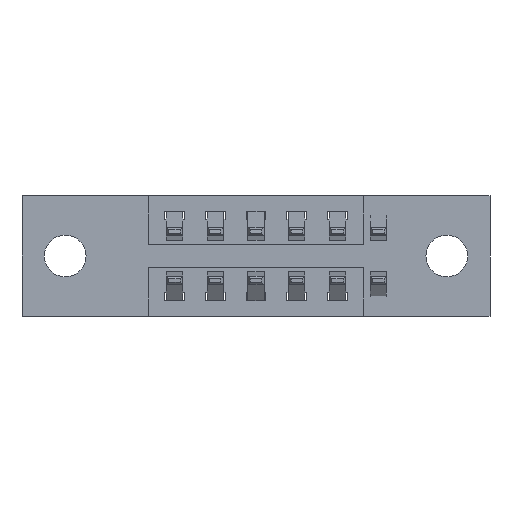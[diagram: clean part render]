
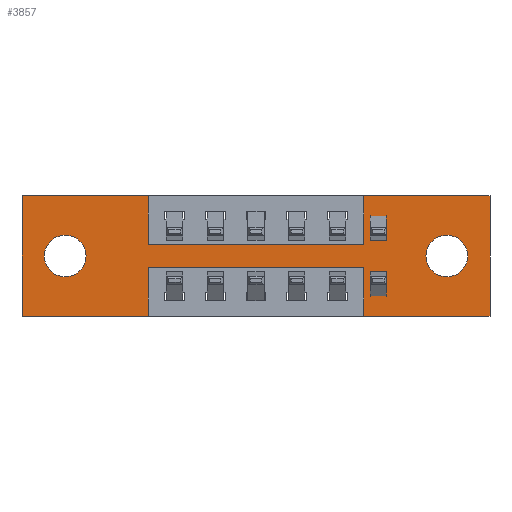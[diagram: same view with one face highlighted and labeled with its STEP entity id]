
A CAD part, front view. The second image highlights one B-rep face of the part: STEP entity #3857.
In plain terms, the highlighted planar face has unit normal (0, -1, 0).
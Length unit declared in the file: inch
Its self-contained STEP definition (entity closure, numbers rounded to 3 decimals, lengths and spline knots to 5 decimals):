
#3 = AXIS2_PLACEMENT_3D ( 'NONE', #1842, #5162, #1243 ) ;
#109 = ORIENTED_EDGE ( 'NONE', *, *, #1768, .F. ) ;
#117 = EDGE_CURVE ( 'NONE', #2051, #4349, #4844, .T. ) ;
#152 = ORIENTED_EDGE ( 'NONE', *, *, #5313, .T. ) ;
#249 = CARTESIAN_POINT ( 'NONE',  ( 0.3875, 0., -0.22 ) ) ;
#291 = DIRECTION ( 'NONE',  ( 0., 0., -1. ) ) ;
#363 = VECTOR ( 'NONE', #3285, 39.37008 ) ;
#412 = VERTEX_POINT ( 'NONE', #2146 ) ;
#483 = EDGE_CURVE ( 'NONE', #7399, #4806, #1431, .T. ) ;
#634 = ORIENTED_EDGE ( 'NONE', *, *, #5431, .F. ) ;
#654 = CARTESIAN_POINT ( 'NONE',  ( 0.3875, 0., 0. ) ) ;
#701 = VECTOR ( 'NONE', #8024, 39.37008 ) ;
#726 = ORIENTED_EDGE ( 'NONE', *, *, #6611, .F. ) ;
#767 = VECTOR ( 'NONE', #4668, 39.37008 ) ;
#812 = ORIENTED_EDGE ( 'NONE', *, *, #483, .F. ) ;
#901 = VERTEX_POINT ( 'NONE', #5119 ) ;
#937 = FACE_BOUND ( 'NONE', #2978, .T. ) ;
#973 = DIRECTION ( 'NONE',  ( -1., 0., 0. ) ) ;
#976 = VERTEX_POINT ( 'NONE', #654 ) ;
#1032 = LINE ( 'NONE', #2331, #8060 ) ;
#1066 = DIRECTION ( 'NONE',  ( 1., 0., 0. ) ) ;
#1097 = CARTESIAN_POINT ( 'NONE',  ( 1.0475, 0., -0.37 ) ) ;
#1143 = DIRECTION ( 'NONE',  ( 0., 1., 0. ) ) ;
#1144 = ORIENTED_EDGE ( 'NONE', *, *, #7149, .F. ) ;
#1153 = AXIS2_PLACEMENT_3D ( 'NONE', #3243, #4054, #6371 ) ;
#1190 = ORIENTED_EDGE ( 'NONE', *, *, #117, .F. ) ;
#1243 = DIRECTION ( 'NONE',  ( 0., 0., 1. ) ) ;
#1252 = EDGE_CURVE ( 'NONE', #3154, #3915, #2502, .T. ) ;
#1256 = DIRECTION ( 'NONE',  ( 0., 0., -1. ) ) ;
#1431 = LINE ( 'NONE', #4754, #701 ) ;
#1496 = LINE ( 'NONE', #6667, #3883 ) ;
#1506 = ORIENTED_EDGE ( 'NONE', *, *, #5541, .F. ) ;
#1603 = AXIS2_PLACEMENT_3D ( 'NONE', #4705, #3574, #291 ) ;
#1697 = CARTESIAN_POINT ( 'NONE',  ( 0.1325, 0., -0.185 ) ) ;
#1721 = EDGE_CURVE ( 'NONE', #2706, #2051, #1496, .T. ) ;
#1768 = EDGE_CURVE ( 'NONE', #976, #3020, #8307, .T. ) ;
#1842 = CARTESIAN_POINT ( 'NONE',  ( 0.1325, 0., -0.185 ) ) ;
#1912 = CIRCLE ( 'NONE', #7168, 0.064 ) ;
#2051 = VERTEX_POINT ( 'NONE', #7431 ) ;
#2075 = LINE ( 'NONE', #3573, #767 ) ;
#2146 = CARTESIAN_POINT ( 'NONE',  ( 1.435, 0., 0. ) ) ;
#2331 = CARTESIAN_POINT ( 'NONE',  ( 0.3875, 0., -0.15 ) ) ;
#2340 = CARTESIAN_POINT ( 'NONE',  ( 0.3875, 0., 0. ) ) ;
#2388 = EDGE_CURVE ( 'NONE', #6549, #412, #3923, .T. ) ;
#2502 = CIRCLE ( 'NONE', #1153, 0.064 ) ;
#2618 = EDGE_CURVE ( 'NONE', #5422, #976, #2075, .T. ) ;
#2706 = VERTEX_POINT ( 'NONE', #1097 ) ;
#2717 = EDGE_CURVE ( 'NONE', #4806, #5422, #3703, .T. ) ;
#2735 = CIRCLE ( 'NONE', #6130, 0.064 ) ;
#2783 = ORIENTED_EDGE ( 'NONE', *, *, #3291, .F. ) ;
#2978 = EDGE_LOOP ( 'NONE', ( #4684, #8267 ) ) ;
#3020 = VERTEX_POINT ( 'NONE', #7974 ) ;
#3055 = DIRECTION ( 'NONE',  ( 0., 0., 1. ) ) ;
#3154 = VERTEX_POINT ( 'NONE', #4916 ) ;
#3180 = CARTESIAN_POINT ( 'NONE',  ( 0.3875, 0., -0.37 ) ) ;
#3207 = VERTEX_POINT ( 'NONE', #3937 ) ;
#3243 = CARTESIAN_POINT ( 'NONE',  ( 1.3025, 0., -0.185 ) ) ;
#3285 = DIRECTION ( 'NONE',  ( 1., 0., 0. ) ) ;
#3291 = EDGE_CURVE ( 'NONE', #7271, #6549, #6526, .T. ) ;
#3311 = CARTESIAN_POINT ( 'NONE',  ( 1.3025, 0., -0.185 ) ) ;
#3351 = DIRECTION ( 'NONE',  ( 0., 0., -1. ) ) ;
#3374 = CARTESIAN_POINT ( 'NONE',  ( 1.0475, 0., 0. ) ) ;
#3527 = FACE_BOUND ( 'NONE', #5461, .T. ) ;
#3556 = VECTOR ( 'NONE', #7145, 39.37008 ) ;
#3573 = CARTESIAN_POINT ( 'NONE',  ( 0., 0., 0. ) ) ;
#3574 = DIRECTION ( 'NONE',  ( 0., -1., 0. ) ) ;
#3621 = CARTESIAN_POINT ( 'NONE',  ( 1.0475, 0., 0. ) ) ;
#3690 = VECTOR ( 'NONE', #6161, 39.37008 ) ;
#3703 = LINE ( 'NONE', #4426, #7546 ) ;
#3704 = CARTESIAN_POINT ( 'NONE',  ( 1.3025, 0., -0.249 ) ) ;
#3734 = ORIENTED_EDGE ( 'NONE', *, *, #2388, .F. ) ;
#3857 = ADVANCED_FACE ( 'NONE', ( #937, #3527, #5542 ), #6764, .T. ) ;
#3883 = VECTOR ( 'NONE', #8043, 39.37008 ) ;
#3891 = ORIENTED_EDGE ( 'NONE', *, *, #6278, .T. ) ;
#3915 = VERTEX_POINT ( 'NONE', #3704 ) ;
#3923 = LINE ( 'NONE', #4004, #363 ) ;
#3937 = CARTESIAN_POINT ( 'NONE',  ( 1.435, 0., -0.37 ) ) ;
#3999 = CARTESIAN_POINT ( 'NONE',  ( 1.435, 0., 0. ) ) ;
#4004 = CARTESIAN_POINT ( 'NONE',  ( 0., 0., 0. ) ) ;
#4054 = DIRECTION ( 'NONE',  ( 0., 1., 0. ) ) ;
#4223 = LINE ( 'NONE', #5488, #7474 ) ;
#4225 = VERTEX_POINT ( 'NONE', #6026 ) ;
#4349 = VERTEX_POINT ( 'NONE', #6268 ) ;
#4426 = CARTESIAN_POINT ( 'NONE',  ( 0., 0., 0. ) ) ;
#4668 = DIRECTION ( 'NONE',  ( 1., 0., 0. ) ) ;
#4684 = ORIENTED_EDGE ( 'NONE', *, *, #1252, .T. ) ;
#4705 = CARTESIAN_POINT ( 'NONE',  ( 0., 0., -0.37 ) ) ;
#4754 = CARTESIAN_POINT ( 'NONE',  ( 0., 0., -0.37 ) ) ;
#4806 = VERTEX_POINT ( 'NONE', #5565 ) ;
#4844 = LINE ( 'NONE', #249, #3690 ) ;
#4900 = CIRCLE ( 'NONE', #3, 0.064 ) ;
#4916 = CARTESIAN_POINT ( 'NONE',  ( 1.3025, 0., -0.121 ) ) ;
#5119 = CARTESIAN_POINT ( 'NONE',  ( 0.1325, 0., -0.249 ) ) ;
#5162 = DIRECTION ( 'NONE',  ( 0., 1., 0. ) ) ;
#5226 = CARTESIAN_POINT ( 'NONE',  ( 0., 0., 0. ) ) ;
#5313 = EDGE_CURVE ( 'NONE', #901, #4225, #1912, .T. ) ;
#5422 = VERTEX_POINT ( 'NONE', #5226 ) ;
#5431 = EDGE_CURVE ( 'NONE', #412, #3207, #8374, .T. ) ;
#5440 = CARTESIAN_POINT ( 'NONE',  ( 1.0475, 0., -0.15 ) ) ;
#5461 = EDGE_LOOP ( 'NONE', ( #3891, #152 ) ) ;
#5488 = CARTESIAN_POINT ( 'NONE',  ( 0., 0., -0.37 ) ) ;
#5541 = EDGE_CURVE ( 'NONE', #3207, #2706, #4223, .T. ) ;
#5542 = FACE_OUTER_BOUND ( 'NONE', #5646, .T. ) ;
#5565 = CARTESIAN_POINT ( 'NONE',  ( 0., 0., -0.37 ) ) ;
#5646 = EDGE_LOOP ( 'NONE', ( #1144, #1190, #8023, #1506, #634, #3734, #2783, #726, #109, #7577, #7629, #812 ) ) ;
#5796 = EDGE_CURVE ( 'NONE', #3915, #3154, #2735, .T. ) ;
#5890 = DIRECTION ( 'NONE',  ( 0., 0., 1. ) ) ;
#6026 = CARTESIAN_POINT ( 'NONE',  ( 0.1325, 0., -0.121 ) ) ;
#6130 = AXIS2_PLACEMENT_3D ( 'NONE', #3311, #8407, #1256 ) ;
#6161 = DIRECTION ( 'NONE',  ( -1., 0., 0. ) ) ;
#6207 = VECTOR ( 'NONE', #5890, 39.37008 ) ;
#6268 = CARTESIAN_POINT ( 'NONE',  ( 0.3875, 0., -0.22 ) ) ;
#6278 = EDGE_CURVE ( 'NONE', #4225, #901, #4900, .T. ) ;
#6371 = DIRECTION ( 'NONE',  ( 0., 0., -1. ) ) ;
#6526 = LINE ( 'NONE', #3374, #6207 ) ;
#6538 = LINE ( 'NONE', #3180, #7503 ) ;
#6549 = VERTEX_POINT ( 'NONE', #3621 ) ;
#6611 = EDGE_CURVE ( 'NONE', #3020, #7271, #1032, .T. ) ;
#6667 = CARTESIAN_POINT ( 'NONE',  ( 1.0475, 0., -0.37 ) ) ;
#6764 = PLANE ( 'NONE',  #1603 ) ;
#6981 = VECTOR ( 'NONE', #7528, 39.37008 ) ;
#7145 = DIRECTION ( 'NONE',  ( 0., 0., -1. ) ) ;
#7149 = EDGE_CURVE ( 'NONE', #4349, #7399, #6538, .T. ) ;
#7168 = AXIS2_PLACEMENT_3D ( 'NONE', #1697, #1143, #8208 ) ;
#7271 = VERTEX_POINT ( 'NONE', #5440 ) ;
#7399 = VERTEX_POINT ( 'NONE', #8191 ) ;
#7431 = CARTESIAN_POINT ( 'NONE',  ( 1.0475, 0., -0.22 ) ) ;
#7474 = VECTOR ( 'NONE', #973, 39.37008 ) ;
#7503 = VECTOR ( 'NONE', #3351, 39.37008 ) ;
#7528 = DIRECTION ( 'NONE',  ( 0., 0., -1. ) ) ;
#7546 = VECTOR ( 'NONE', #3055, 39.37008 ) ;
#7577 = ORIENTED_EDGE ( 'NONE', *, *, #2618, .F. ) ;
#7629 = ORIENTED_EDGE ( 'NONE', *, *, #2717, .F. ) ;
#7974 = CARTESIAN_POINT ( 'NONE',  ( 0.3875, 0., -0.15 ) ) ;
#8023 = ORIENTED_EDGE ( 'NONE', *, *, #1721, .F. ) ;
#8024 = DIRECTION ( 'NONE',  ( -1., 0., 0. ) ) ;
#8043 = DIRECTION ( 'NONE',  ( 0., 0., 1. ) ) ;
#8060 = VECTOR ( 'NONE', #1066, 39.37008 ) ;
#8191 = CARTESIAN_POINT ( 'NONE',  ( 0.3875, 0., -0.37 ) ) ;
#8208 = DIRECTION ( 'NONE',  ( 0., 0., 1. ) ) ;
#8267 = ORIENTED_EDGE ( 'NONE', *, *, #5796, .T. ) ;
#8307 = LINE ( 'NONE', #2340, #6981 ) ;
#8374 = LINE ( 'NONE', #3999, #3556 ) ;
#8407 = DIRECTION ( 'NONE',  ( 0., 1., 0. ) ) ;
